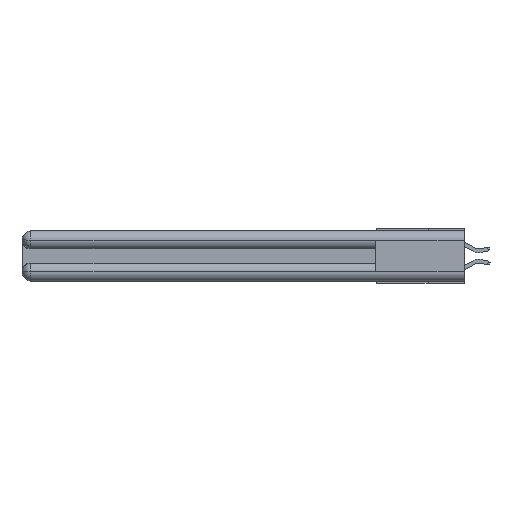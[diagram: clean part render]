
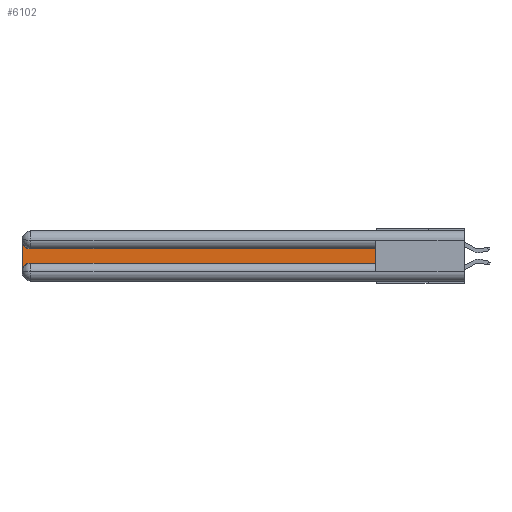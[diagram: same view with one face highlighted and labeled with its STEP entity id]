
A CAD part, left-side view. The second image highlights one B-rep face of the part: STEP entity #6102.
In plain terms, the highlighted planar face has unit normal (-1, 0, 0).
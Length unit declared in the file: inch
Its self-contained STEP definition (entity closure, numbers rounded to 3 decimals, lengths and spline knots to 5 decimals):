
#523 = CARTESIAN_POINT ( 'NONE',  ( 0.075, 0.6, -0.1225 ) ) ;
#617 = ORIENTED_EDGE ( 'NONE', *, *, #28736, .T. ) ;
#1231 = EDGE_CURVE ( 'NONE', #12190, #25720, #17275, .T. ) ;
#2733 = DIRECTION ( 'NONE',  ( 0., 0., -1. ) ) ;
#3294 = CARTESIAN_POINT ( 'NONE',  ( 0.075, 2.94, -0.2775 ) ) ;
#3509 = CARTESIAN_POINT ( 'NONE',  ( 0.075, 3., -0.0625 ) ) ;
#3708 = ORIENTED_EDGE ( 'NONE', *, *, #1231, .T. ) ;
#5485 = ORIENTED_EDGE ( 'NONE', *, *, #22998, .T. ) ;
#5618 = DIRECTION ( 'NONE',  ( 1., 0., 0. ) ) ;
#6102 = ADVANCED_FACE ( 'NONE', ( #28143 ), #7339, .F. ) ;
#6636 = DIRECTION ( 'NONE',  ( 0., 0., -1. ) ) ;
#7078 = CARTESIAN_POINT ( 'NONE',  ( 0.075, 2.94, -0.1225 ) ) ;
#7141 = CARTESIAN_POINT ( 'NONE',  ( 0.075, 0.6, -0.2175 ) ) ;
#7339 = PLANE ( 'NONE',  #16358 ) ;
#7764 = VERTEX_POINT ( 'NONE', #33436 ) ;
#9686 = CARTESIAN_POINT ( 'NONE',  ( 0.075, 3., -0.2175 ) ) ;
#10172 = CARTESIAN_POINT ( 'NONE',  ( 0.075, 3., -0.1225 ) ) ;
#10270 = CIRCLE ( 'NONE', #30838, 0.06 ) ;
#12190 = VERTEX_POINT ( 'NONE', #31326 ) ;
#12236 = LINE ( 'NONE', #9686, #18800 ) ;
#12335 = DIRECTION ( 'NONE',  ( 1., 0., 0. ) ) ;
#12434 = LINE ( 'NONE', #19264, #22742 ) ;
#13318 = VERTEX_POINT ( 'NONE', #3509 ) ;
#13473 = CARTESIAN_POINT ( 'NONE',  ( 0.075, 0.6, -0.1225 ) ) ;
#16358 = AXIS2_PLACEMENT_3D ( 'NONE', #10172, #23401, #23635 ) ;
#16443 = VECTOR ( 'NONE', #32450, 39.37008 ) ;
#16543 = AXIS2_PLACEMENT_3D ( 'NONE', #3294, #5618, #6636 ) ;
#17275 = LINE ( 'NONE', #30108, #16443 ) ;
#17974 = CARTESIAN_POINT ( 'NONE',  ( 0.075, 2.94, -0.0625 ) ) ;
#18096 = CIRCLE ( 'NONE', #16543, 0.06 ) ;
#18800 = VECTOR ( 'NONE', #33106, 39.37008 ) ;
#19123 = VERTEX_POINT ( 'NONE', #523 ) ;
#19264 = CARTESIAN_POINT ( 'NONE',  ( 0.075, 0.6, -0.2175 ) ) ;
#19972 = ORIENTED_EDGE ( 'NONE', *, *, #20694, .T. ) ;
#20694 = EDGE_CURVE ( 'NONE', #25720, #19123, #12434, .T. ) ;
#22742 = VECTOR ( 'NONE', #27043, 39.37008 ) ;
#22998 = EDGE_CURVE ( 'NONE', #7764, #12190, #18096, .T. ) ;
#23086 = EDGE_LOOP ( 'NONE', ( #25564, #617, #26082, #5485, #3708, #19972 ) ) ;
#23401 = DIRECTION ( 'NONE',  ( 1., 0., 0. ) ) ;
#23635 = DIRECTION ( 'NONE',  ( 0., 0., -1. ) ) ;
#25065 = LINE ( 'NONE', #13473, #26742 ) ;
#25564 = ORIENTED_EDGE ( 'NONE', *, *, #33021, .T. ) ;
#25720 = VERTEX_POINT ( 'NONE', #7141 ) ;
#26082 = ORIENTED_EDGE ( 'NONE', *, *, #33722, .T. ) ;
#26742 = VECTOR ( 'NONE', #29505, 39.37008 ) ;
#27043 = DIRECTION ( 'NONE',  ( 0., 0., 1. ) ) ;
#28143 = FACE_OUTER_BOUND ( 'NONE', #23086, .T. ) ;
#28736 = EDGE_CURVE ( 'NONE', #29133, #13318, #10270, .T. ) ;
#29133 = VERTEX_POINT ( 'NONE', #7078 ) ;
#29505 = DIRECTION ( 'NONE',  ( 0., 1., 0. ) ) ;
#30108 = CARTESIAN_POINT ( 'NONE',  ( 0.075, 0.6, -0.2175 ) ) ;
#30838 = AXIS2_PLACEMENT_3D ( 'NONE', #17974, #12335, #2733 ) ;
#31326 = CARTESIAN_POINT ( 'NONE',  ( 0.075, 2.94, -0.2175 ) ) ;
#32450 = DIRECTION ( 'NONE',  ( 0., -1., 0. ) ) ;
#33021 = EDGE_CURVE ( 'NONE', #19123, #29133, #25065, .T. ) ;
#33106 = DIRECTION ( 'NONE',  ( 0., 0., -1. ) ) ;
#33436 = CARTESIAN_POINT ( 'NONE',  ( 0.075, 3., -0.2775 ) ) ;
#33722 = EDGE_CURVE ( 'NONE', #13318, #7764, #12236, .T. ) ;
